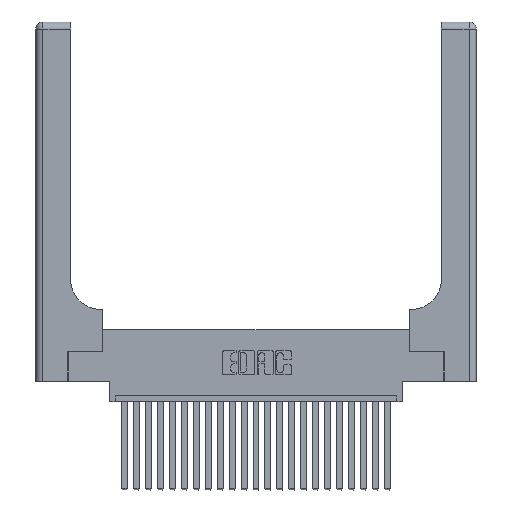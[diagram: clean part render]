
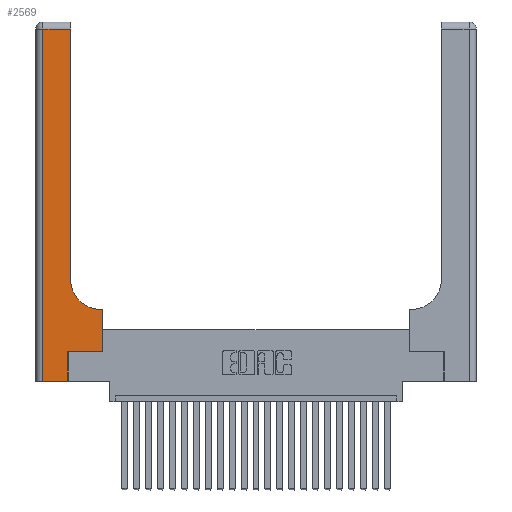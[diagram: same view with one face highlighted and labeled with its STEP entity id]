
A CAD part, top view. The second image highlights one B-rep face of the part: STEP entity #2569.
In plain terms, the highlighted planar face has unit normal (0, 0, 1).
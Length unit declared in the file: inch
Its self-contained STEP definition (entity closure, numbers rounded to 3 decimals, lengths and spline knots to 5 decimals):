
#7 = EDGE_CURVE ( 'NONE', #14419, #10625, #20090, .T. ) ;
#616 = VERTEX_POINT ( 'NONE', #20166 ) ;
#626 = EDGE_CURVE ( 'NONE', #13625, #616, #12586, .T. ) ;
#2073 = ORIENTED_EDGE ( 'NONE', *, *, #9080, .T. ) ;
#2137 = EDGE_CURVE ( 'NONE', #5670, #13625, #2967, .T. ) ;
#2394 = LINE ( 'NONE', #16003, #16862 ) ;
#2401 = DIRECTION ( 'NONE',  ( -1., 0., 0. ) ) ;
#2569 = ADVANCED_FACE ( 'NONE', ( #24667 ), #20093, .F. ) ;
#2967 = LINE ( 'NONE', #3243, #5668 ) ;
#3243 = CARTESIAN_POINT ( 'NONE',  ( 0.269, 0.25, 0.37 ) ) ;
#4627 = EDGE_LOOP ( 'NONE', ( #21682, #17017, #12657, #2073, #21372, #7065, #10725, #5226, #11769 ) ) ;
#4858 = CARTESIAN_POINT ( 'NONE',  ( 0., 3., 0.37 ) ) ;
#4883 = DIRECTION ( 'NONE',  ( 0., -1., 0. ) ) ;
#5226 = ORIENTED_EDGE ( 'NONE', *, *, #12215, .T. ) ;
#5352 = DIRECTION ( 'NONE',  ( 0., 1., 0. ) ) ;
#5668 = VECTOR ( 'NONE', #16269, 39.37008 ) ;
#5670 = VERTEX_POINT ( 'NONE', #6395 ) ;
#6003 = VECTOR ( 'NONE', #5352, 39.37008 ) ;
#6190 = DIRECTION ( 'NONE',  ( -1., 0., 0. ) ) ;
#6395 = CARTESIAN_POINT ( 'NONE',  ( 0.269, 0.25, 0.37 ) ) ;
#6562 = VECTOR ( 'NONE', #10949, 39.37008 ) ;
#6817 = CARTESIAN_POINT ( 'NONE',  ( 0.5415, 0.6, 0.37 ) ) ;
#6896 = VERTEX_POINT ( 'NONE', #13083 ) ;
#7065 = ORIENTED_EDGE ( 'NONE', *, *, #2137, .T. ) ;
#7132 = LINE ( 'NONE', #11550, #17354 ) ;
#8834 = CARTESIAN_POINT ( 'NONE',  ( 0.269, 0., 0.37 ) ) ;
#8946 = CARTESIAN_POINT ( 'NONE',  ( 0.269, 0., 0.37 ) ) ;
#9080 = EDGE_CURVE ( 'NONE', #6896, #12417, #11881, .T. ) ;
#9192 = CARTESIAN_POINT ( 'NONE',  ( 0.5415, 0.85, 0.37 ) ) ;
#9455 = DIRECTION ( 'NONE',  ( 0., 0., -1. ) ) ;
#9686 = VECTOR ( 'NONE', #2401, 39.37008 ) ;
#9700 = EDGE_CURVE ( 'NONE', #13996, #6896, #18211, .T. ) ;
#9719 = DIRECTION ( 'NONE',  ( 0., 1., 0. ) ) ;
#9773 = VECTOR ( 'NONE', #4883, 39.37008 ) ;
#9809 = CARTESIAN_POINT ( 'NONE',  ( 0.2915, 0.6, 0.37 ) ) ;
#10625 = VERTEX_POINT ( 'NONE', #14798 ) ;
#10725 = ORIENTED_EDGE ( 'NONE', *, *, #626, .T. ) ;
#10830 = CARTESIAN_POINT ( 'NONE',  ( 0.06, 3., 0.37 ) ) ;
#10949 = DIRECTION ( 'NONE',  ( 0., 1., 0. ) ) ;
#11207 = AXIS2_PLACEMENT_3D ( 'NONE', #9192, #14875, #18947 ) ;
#11550 = CARTESIAN_POINT ( 'NONE',  ( 0.2915, 3., 0.37 ) ) ;
#11769 = ORIENTED_EDGE ( 'NONE', *, *, #7, .T. ) ;
#11881 = LINE ( 'NONE', #23612, #13385 ) ;
#12215 = EDGE_CURVE ( 'NONE', #616, #14419, #14786, .T. ) ;
#12417 = VERTEX_POINT ( 'NONE', #8834 ) ;
#12586 = LINE ( 'NONE', #22169, #6003 ) ;
#12657 = ORIENTED_EDGE ( 'NONE', *, *, #9700, .T. ) ;
#13083 = CARTESIAN_POINT ( 'NONE',  ( 0.06, 0., 0.37 ) ) ;
#13385 = VECTOR ( 'NONE', #17954, 39.37008 ) ;
#13625 = VERTEX_POINT ( 'NONE', #21431 ) ;
#13712 = LINE ( 'NONE', #8946, #6562 ) ;
#13996 = VERTEX_POINT ( 'NONE', #20744 ) ;
#14419 = VERTEX_POINT ( 'NONE', #6817 ) ;
#14786 = LINE ( 'NONE', #9809, #9686 ) ;
#14798 = CARTESIAN_POINT ( 'NONE',  ( 0.2915, 0.85, 0.37 ) ) ;
#14875 = DIRECTION ( 'NONE',  ( 0., 0., -1. ) ) ;
#15182 = DIRECTION ( 'NONE',  ( -1., 0., 0. ) ) ;
#16003 = CARTESIAN_POINT ( 'NONE',  ( 0., 2.94, 0.37 ) ) ;
#16269 = DIRECTION ( 'NONE',  ( 1., 0., 0. ) ) ;
#16396 = AXIS2_PLACEMENT_3D ( 'NONE', #4858, #9455, #15182 ) ;
#16862 = VECTOR ( 'NONE', #6190, 39.37008 ) ;
#17017 = ORIENTED_EDGE ( 'NONE', *, *, #21396, .T. ) ;
#17354 = VECTOR ( 'NONE', #9719, 39.37008 ) ;
#17954 = DIRECTION ( 'NONE',  ( 1., 0., 0. ) ) ;
#18211 = LINE ( 'NONE', #10830, #9773 ) ;
#18947 = DIRECTION ( 'NONE',  ( 1., 0., 0. ) ) ;
#20090 = CIRCLE ( 'NONE', #11207, 0.25 ) ;
#20093 = PLANE ( 'NONE',  #16396 ) ;
#20166 = CARTESIAN_POINT ( 'NONE',  ( 0.5585, 0.6, 0.37 ) ) ;
#20744 = CARTESIAN_POINT ( 'NONE',  ( 0.06, 2.94, 0.37 ) ) ;
#21372 = ORIENTED_EDGE ( 'NONE', *, *, #22605, .T. ) ;
#21396 = EDGE_CURVE ( 'NONE', #22738, #13996, #2394, .T. ) ;
#21431 = CARTESIAN_POINT ( 'NONE',  ( 0.5585, 0.25, 0.37 ) ) ;
#21682 = ORIENTED_EDGE ( 'NONE', *, *, #23359, .T. ) ;
#22169 = CARTESIAN_POINT ( 'NONE',  ( 0.5585, 0.25, 0.37 ) ) ;
#22605 = EDGE_CURVE ( 'NONE', #12417, #5670, #13712, .T. ) ;
#22738 = VERTEX_POINT ( 'NONE', #22987 ) ;
#22987 = CARTESIAN_POINT ( 'NONE',  ( 0.2915, 2.94, 0.37 ) ) ;
#23359 = EDGE_CURVE ( 'NONE', #10625, #22738, #7132, .T. ) ;
#23612 = CARTESIAN_POINT ( 'NONE',  ( 0., 0., 0.37 ) ) ;
#24667 = FACE_OUTER_BOUND ( 'NONE', #4627, .T. ) ;
